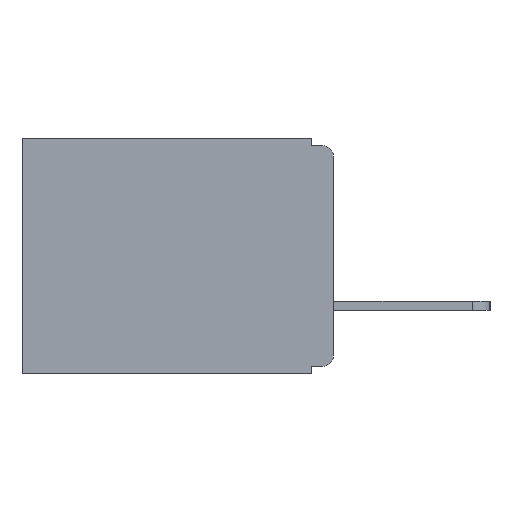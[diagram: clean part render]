
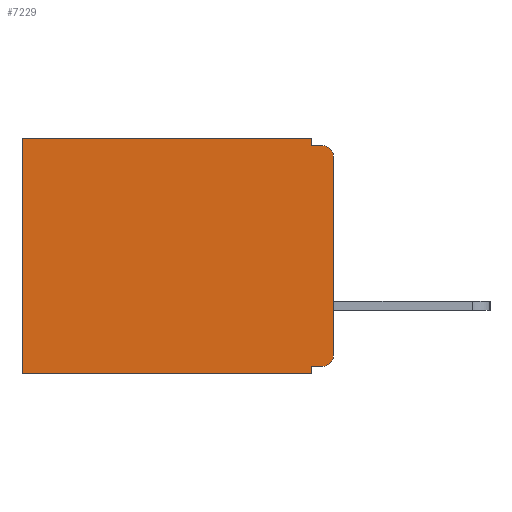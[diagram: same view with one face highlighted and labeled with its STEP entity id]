
A CAD part, left-side view. The second image highlights one B-rep face of the part: STEP entity #7229.
In plain terms, the highlighted planar face has unit normal (-1, 0, 0).
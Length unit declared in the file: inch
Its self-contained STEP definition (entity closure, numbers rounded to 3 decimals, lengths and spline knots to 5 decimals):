
#25 = CARTESIAN_POINT ( 'NONE',  ( 0.3, 0.015, -0.025 ) ) ;
#421 = VECTOR ( 'NONE', #4624, 39.37008 ) ;
#546 = ORIENTED_EDGE ( 'NONE', *, *, #10006, .F. ) ;
#592 = CARTESIAN_POINT ( 'NONE',  ( 0.3, 0.015, -0.01 ) ) ;
#1156 = EDGE_LOOP ( 'NONE', ( #2908, #4547, #546, #16786, #3287, #21805, #4049, #2687, #13170, #18519 ) ) ;
#1513 = CARTESIAN_POINT ( 'NONE',  ( 0.3, 0., -0.33 ) ) ;
#1633 = VERTEX_POINT ( 'NONE', #6551 ) ;
#1802 = DIRECTION ( 'NONE',  ( 0., 0., -1. ) ) ;
#2197 = CARTESIAN_POINT ( 'NONE',  ( 0.3, 0., -0.32 ) ) ;
#2570 = EDGE_CURVE ( 'NONE', #12651, #5450, #13433, .T. ) ;
#2687 = ORIENTED_EDGE ( 'NONE', *, *, #2570, .F. ) ;
#2880 = CARTESIAN_POINT ( 'NONE',  ( 0.3, 0., -0.33 ) ) ;
#2908 = ORIENTED_EDGE ( 'NONE', *, *, #19806, .F. ) ;
#3212 = DIRECTION ( 'NONE',  ( 0., 0., -1. ) ) ;
#3287 = ORIENTED_EDGE ( 'NONE', *, *, #15935, .T. ) ;
#3345 = LINE ( 'NONE', #8678, #16330 ) ;
#3783 = VECTOR ( 'NONE', #3212, 39.37008 ) ;
#3917 = VECTOR ( 'NONE', #4399, 39.37008 ) ;
#3964 = DIRECTION ( 'NONE',  ( 0., 1., 0. ) ) ;
#4049 = ORIENTED_EDGE ( 'NONE', *, *, #10229, .F. ) ;
#4050 = VERTEX_POINT ( 'NONE', #8685 ) ;
#4372 = FACE_OUTER_BOUND ( 'NONE', #1156, .T. ) ;
#4397 = DIRECTION ( 'NONE',  ( 0., -1., 0. ) ) ;
#4399 = DIRECTION ( 'NONE',  ( 0., 0., -1. ) ) ;
#4547 = ORIENTED_EDGE ( 'NONE', *, *, #8592, .T. ) ;
#4624 = DIRECTION ( 'NONE',  ( 0., 0., -1. ) ) ;
#5102 = AXIS2_PLACEMENT_3D ( 'NONE', #12433, #11803, #11755 ) ;
#5450 = VERTEX_POINT ( 'NONE', #6267 ) ;
#5525 = EDGE_CURVE ( 'NONE', #1633, #13672, #21382, .T. ) ;
#5987 = VECTOR ( 'NONE', #15082, 39.37008 ) ;
#6267 = CARTESIAN_POINT ( 'NONE',  ( 0.3, 0.031, -0.33 ) ) ;
#6551 = CARTESIAN_POINT ( 'NONE',  ( 0.3, 0.015, -0.32 ) ) ;
#6803 = LINE ( 'NONE', #16139, #10218 ) ;
#6833 = AXIS2_PLACEMENT_3D ( 'NONE', #25, #11991, #1802 ) ;
#7229 = ADVANCED_FACE ( 'NONE', ( #4372 ), #11231, .F. ) ;
#8381 = LINE ( 'NONE', #19516, #21311 ) ;
#8592 = EDGE_CURVE ( 'NONE', #13409, #13431, #15122, .T. ) ;
#8678 = CARTESIAN_POINT ( 'NONE',  ( 0.3, 0.437, -0.33 ) ) ;
#8685 = CARTESIAN_POINT ( 'NONE',  ( 0.3, 0.031, 0. ) ) ;
#9103 = EDGE_CURVE ( 'NONE', #12914, #17418, #3345, .T. ) ;
#9306 = VECTOR ( 'NONE', #3964, 39.37008 ) ;
#9414 = DIRECTION ( 'NONE',  ( 0., 1., 0. ) ) ;
#9547 = LINE ( 'NONE', #2880, #421 ) ;
#9986 = CARTESIAN_POINT ( 'NONE',  ( 0.3, 0.031, 0. ) ) ;
#10006 = EDGE_CURVE ( 'NONE', #14382, #13431, #6803, .T. ) ;
#10137 = DIRECTION ( 'NONE',  ( 0., 0., -1. ) ) ;
#10203 = CARTESIAN_POINT ( 'NONE',  ( 0.3, 0.031, -0.01 ) ) ;
#10210 = CARTESIAN_POINT ( 'NONE',  ( 0.3, 0.031, -0.32 ) ) ;
#10218 = VECTOR ( 'NONE', #4397, 39.37008 ) ;
#10229 = EDGE_CURVE ( 'NONE', #5450, #17418, #20000, .T. ) ;
#10338 = DIRECTION ( 'NONE',  ( -1., 0., 0. ) ) ;
#10352 = CARTESIAN_POINT ( 'NONE',  ( 0.3, 0.015, -0.305 ) ) ;
#10416 = CARTESIAN_POINT ( 'NONE',  ( 0.3, 0.437, -0.33 ) ) ;
#11231 = PLANE ( 'NONE',  #5102 ) ;
#11755 = DIRECTION ( 'NONE',  ( 0., 0., -1. ) ) ;
#11803 = DIRECTION ( 'NONE',  ( 1., 0., 0. ) ) ;
#11991 = DIRECTION ( 'NONE',  ( -1., 0., 0. ) ) ;
#12433 = CARTESIAN_POINT ( 'NONE',  ( 0.3, 0., -0.33 ) ) ;
#12651 = VERTEX_POINT ( 'NONE', #10210 ) ;
#12914 = VERTEX_POINT ( 'NONE', #15869 ) ;
#13170 = ORIENTED_EDGE ( 'NONE', *, *, #19577, .F. ) ;
#13175 = CARTESIAN_POINT ( 'NONE',  ( 0.3, 0., -0.305 ) ) ;
#13409 = VERTEX_POINT ( 'NONE', #20969 ) ;
#13431 = VERTEX_POINT ( 'NONE', #592 ) ;
#13433 = LINE ( 'NONE', #17780, #3917 ) ;
#13672 = VERTEX_POINT ( 'NONE', #13175 ) ;
#14382 = VERTEX_POINT ( 'NONE', #10203 ) ;
#15082 = DIRECTION ( 'NONE',  ( 0., 1., 0. ) ) ;
#15122 = CIRCLE ( 'NONE', #6833, 0.015 ) ;
#15869 = CARTESIAN_POINT ( 'NONE',  ( 0.3, 0.437, 0. ) ) ;
#15935 = EDGE_CURVE ( 'NONE', #4050, #12914, #8381, .T. ) ;
#16139 = CARTESIAN_POINT ( 'NONE',  ( 0.3, 0., -0.01 ) ) ;
#16330 = VECTOR ( 'NONE', #20488, 39.37008 ) ;
#16786 = ORIENTED_EDGE ( 'NONE', *, *, #17238, .F. ) ;
#17238 = EDGE_CURVE ( 'NONE', #4050, #14382, #21247, .T. ) ;
#17418 = VERTEX_POINT ( 'NONE', #10416 ) ;
#17780 = CARTESIAN_POINT ( 'NONE',  ( 0.3, 0.031, -0.33 ) ) ;
#18273 = LINE ( 'NONE', #2197, #9306 ) ;
#18519 = ORIENTED_EDGE ( 'NONE', *, *, #5525, .T. ) ;
#19372 = AXIS2_PLACEMENT_3D ( 'NONE', #10352, #10338, #10137 ) ;
#19516 = CARTESIAN_POINT ( 'NONE',  ( 0.3, 0., 0. ) ) ;
#19577 = EDGE_CURVE ( 'NONE', #1633, #12651, #18273, .T. ) ;
#19806 = EDGE_CURVE ( 'NONE', #13409, #13672, #9547, .T. ) ;
#20000 = LINE ( 'NONE', #1513, #5987 ) ;
#20488 = DIRECTION ( 'NONE',  ( 0., 0., -1. ) ) ;
#20969 = CARTESIAN_POINT ( 'NONE',  ( 0.3, 0., -0.025 ) ) ;
#21247 = LINE ( 'NONE', #9986, #3783 ) ;
#21311 = VECTOR ( 'NONE', #9414, 39.37008 ) ;
#21382 = CIRCLE ( 'NONE', #19372, 0.015 ) ;
#21805 = ORIENTED_EDGE ( 'NONE', *, *, #9103, .T. ) ;
